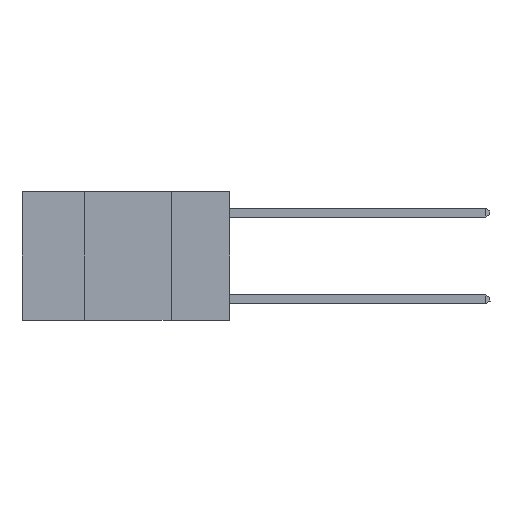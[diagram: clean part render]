
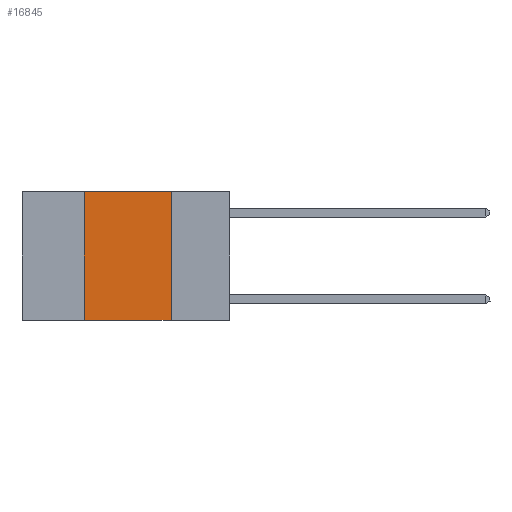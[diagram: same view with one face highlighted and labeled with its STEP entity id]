
A CAD part, left-side view. The second image highlights one B-rep face of the part: STEP entity #16845.
In plain terms, the highlighted planar face has unit normal (-1, 0, 0).
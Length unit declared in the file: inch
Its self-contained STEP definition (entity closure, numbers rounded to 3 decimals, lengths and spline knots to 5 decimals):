
#523 = CARTESIAN_POINT ( 'NONE',  ( 0., 0.6, 0. ) ) ;
#751 = EDGE_LOOP ( 'NONE', ( #5768, #19548, #10894, #20054 ) ) ;
#835 = VECTOR ( 'NONE', #21041, 39.37008 ) ;
#2310 = DIRECTION ( 'NONE',  ( 0., 0., -1. ) ) ;
#3397 = EDGE_CURVE ( 'NONE', #4249, #14123, #6513, .T. ) ;
#3414 = CARTESIAN_POINT ( 'NONE',  ( 0., 0.17, 0. ) ) ;
#3697 = EDGE_CURVE ( 'NONE', #7738, #14123, #18367, .T. ) ;
#4249 = VERTEX_POINT ( 'NONE', #13464 ) ;
#4886 = LINE ( 'NONE', #20573, #13531 ) ;
#4969 = AXIS2_PLACEMENT_3D ( 'NONE', #523, #12642, #2310 ) ;
#5273 = CARTESIAN_POINT ( 'NONE',  ( 0., 0.17, -0.37 ) ) ;
#5768 = ORIENTED_EDGE ( 'NONE', *, *, #3697, .F. ) ;
#6513 = LINE ( 'NONE', #21630, #10563 ) ;
#7738 = VERTEX_POINT ( 'NONE', #3414 ) ;
#9195 = VECTOR ( 'NONE', #22378, 39.37008 ) ;
#9254 = VERTEX_POINT ( 'NONE', #20353 ) ;
#9332 = EDGE_CURVE ( 'NONE', #4249, #9254, #4886, .T. ) ;
#10563 = VECTOR ( 'NONE', #13051, 39.37008 ) ;
#10894 = ORIENTED_EDGE ( 'NONE', *, *, #9332, .F. ) ;
#12642 = DIRECTION ( 'NONE',  ( 1., 0., 0. ) ) ;
#13051 = DIRECTION ( 'NONE',  ( 0., -1., 0. ) ) ;
#13464 = CARTESIAN_POINT ( 'NONE',  ( 0., 0.42, -0.37 ) ) ;
#13531 = VECTOR ( 'NONE', #22322, 39.37008 ) ;
#14123 = VERTEX_POINT ( 'NONE', #5273 ) ;
#14130 = CARTESIAN_POINT ( 'NONE',  ( 0., 0.6, 0. ) ) ;
#14641 = LINE ( 'NONE', #14130, #835 ) ;
#14667 = FACE_OUTER_BOUND ( 'NONE', #751, .T. ) ;
#15520 = CARTESIAN_POINT ( 'NONE',  ( 0., 0.17, 0. ) ) ;
#16039 = PLANE ( 'NONE',  #4969 ) ;
#16845 = ADVANCED_FACE ( 'NONE', ( #14667 ), #16039, .F. ) ;
#18367 = LINE ( 'NONE', #15520, #9195 ) ;
#19548 = ORIENTED_EDGE ( 'NONE', *, *, #20584, .F. ) ;
#20054 = ORIENTED_EDGE ( 'NONE', *, *, #3397, .T. ) ;
#20353 = CARTESIAN_POINT ( 'NONE',  ( 0., 0.42, 0. ) ) ;
#20573 = CARTESIAN_POINT ( 'NONE',  ( 0., 0.42, 0. ) ) ;
#20584 = EDGE_CURVE ( 'NONE', #9254, #7738, #14641, .T. ) ;
#21041 = DIRECTION ( 'NONE',  ( 0., -1., 0. ) ) ;
#21630 = CARTESIAN_POINT ( 'NONE',  ( 0., 0.6, -0.37 ) ) ;
#22322 = DIRECTION ( 'NONE',  ( 0., 0., 1. ) ) ;
#22378 = DIRECTION ( 'NONE',  ( 0., 0., -1. ) ) ;
